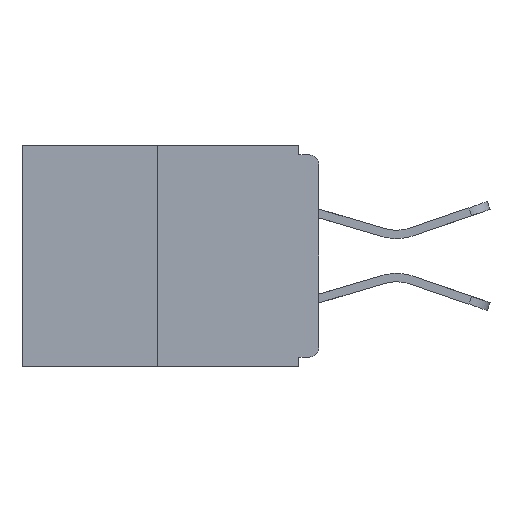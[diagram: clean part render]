
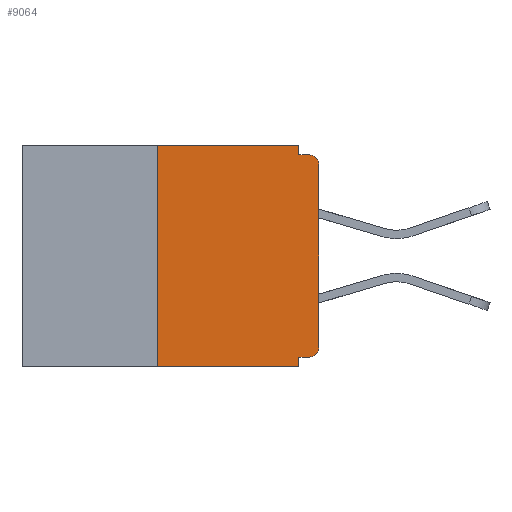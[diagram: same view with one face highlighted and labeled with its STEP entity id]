
A CAD part, left-side view. The second image highlights one B-rep face of the part: STEP entity #9064.
In plain terms, the highlighted planar face has unit normal (-1, 0, 0).
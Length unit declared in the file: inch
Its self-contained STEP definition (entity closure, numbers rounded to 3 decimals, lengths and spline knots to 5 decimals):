
#79 = VECTOR ( 'NONE', #12660, 39.37008 ) ;
#108 = VERTEX_POINT ( 'NONE', #13360 ) ;
#824 = EDGE_CURVE ( 'NONE', #8475, #1453, #8395, .T. ) ;
#834 = VERTEX_POINT ( 'NONE', #13838 ) ;
#1170 = AXIS2_PLACEMENT_3D ( 'NONE', #12093, #9109, #7771 ) ;
#1222 = DIRECTION ( 'NONE',  ( 0., 0., -1. ) ) ;
#1316 = LINE ( 'NONE', #3704, #11945 ) ;
#1453 = VERTEX_POINT ( 'NONE', #11990 ) ;
#1483 = LINE ( 'NONE', #13181, #8561 ) ;
#1779 = VERTEX_POINT ( 'NONE', #2282 ) ;
#2138 = EDGE_CURVE ( 'NONE', #9694, #13709, #9196, .T. ) ;
#2282 = CARTESIAN_POINT ( 'NONE',  ( 0., 0.031, 0. ) ) ;
#2665 = CARTESIAN_POINT ( 'NONE',  ( 0., 0.25, 0. ) ) ;
#2887 = VERTEX_POINT ( 'NONE', #2665 ) ;
#3097 = CIRCLE ( 'NONE', #13831, 0.015 ) ;
#3277 = EDGE_CURVE ( 'NONE', #10018, #8149, #6022, .T. ) ;
#3427 = LINE ( 'NONE', #7977, #13079 ) ;
#3610 = DIRECTION ( 'NONE',  ( -1., 0., 0. ) ) ;
#3704 = CARTESIAN_POINT ( 'NONE',  ( 0., 0.46, 0. ) ) ;
#4407 = CARTESIAN_POINT ( 'NONE',  ( 0., 0.031, -0.343 ) ) ;
#4533 = EDGE_CURVE ( 'NONE', #1779, #9694, #1483, .T. ) ;
#4693 = CARTESIAN_POINT ( 'NONE',  ( 0., 0., -0.03 ) ) ;
#4867 = DIRECTION ( 'NONE',  ( 0., 0., -1. ) ) ;
#5077 = ORIENTED_EDGE ( 'NONE', *, *, #824, .T. ) ;
#5130 = EDGE_CURVE ( 'NONE', #834, #10018, #3097, .T. ) ;
#5134 = CARTESIAN_POINT ( 'NONE',  ( 0., 0., -0.015 ) ) ;
#5145 = VECTOR ( 'NONE', #9404, 39.37008 ) ;
#5468 = LINE ( 'NONE', #6390, #8571 ) ;
#5552 = CARTESIAN_POINT ( 'NONE',  ( 0., 0.031, -0.015 ) ) ;
#5947 = DIRECTION ( 'NONE',  ( 0., 0., 1. ) ) ;
#6022 = LINE ( 'NONE', #10296, #7125 ) ;
#6390 = CARTESIAN_POINT ( 'NONE',  ( 0., 0., -0.328 ) ) ;
#6522 = EDGE_CURVE ( 'NONE', #8149, #13709, #8382, .T. ) ;
#6644 = DIRECTION ( 'NONE',  ( 0., 0., -1. ) ) ;
#6874 = EDGE_CURVE ( 'NONE', #2887, #1779, #1316, .T. ) ;
#6895 = EDGE_CURVE ( 'NONE', #8475, #2887, #3427, .T. ) ;
#7092 = ORIENTED_EDGE ( 'NONE', *, *, #5130, .T. ) ;
#7105 = DIRECTION ( 'NONE',  ( -1., 0., 0. ) ) ;
#7125 = VECTOR ( 'NONE', #5947, 39.37008 ) ;
#7231 = ORIENTED_EDGE ( 'NONE', *, *, #6874, .F. ) ;
#7608 = ORIENTED_EDGE ( 'NONE', *, *, #4533, .F. ) ;
#7771 = DIRECTION ( 'NONE',  ( 0., 0., -1. ) ) ;
#7909 = FACE_OUTER_BOUND ( 'NONE', #12830, .T. ) ;
#7945 = CARTESIAN_POINT ( 'NONE',  ( 0., 0.015, -0.313 ) ) ;
#7977 = CARTESIAN_POINT ( 'NONE',  ( 0., 0.25, 0. ) ) ;
#8149 = VERTEX_POINT ( 'NONE', #4693 ) ;
#8271 = CARTESIAN_POINT ( 'NONE',  ( 0., 0.25, -0.343 ) ) ;
#8382 = CIRCLE ( 'NONE', #11055, 0.015 ) ;
#8395 = LINE ( 'NONE', #10496, #79 ) ;
#8475 = VERTEX_POINT ( 'NONE', #8271 ) ;
#8561 = VECTOR ( 'NONE', #11976, 39.37008 ) ;
#8571 = VECTOR ( 'NONE', #10665, 39.37008 ) ;
#9064 = ADVANCED_FACE ( 'NONE', ( #7909 ), #9875, .F. ) ;
#9109 = DIRECTION ( 'NONE',  ( 1., 0., 0. ) ) ;
#9196 = LINE ( 'NONE', #5134, #5145 ) ;
#9392 = ORIENTED_EDGE ( 'NONE', *, *, #6895, .F. ) ;
#9404 = DIRECTION ( 'NONE',  ( 0., -1., 0. ) ) ;
#9694 = VERTEX_POINT ( 'NONE', #5552 ) ;
#9875 = PLANE ( 'NONE',  #1170 ) ;
#10010 = ORIENTED_EDGE ( 'NONE', *, *, #10137, .F. ) ;
#10018 = VERTEX_POINT ( 'NONE', #12684 ) ;
#10080 = DIRECTION ( 'NONE',  ( 0., 0., 1. ) ) ;
#10137 = EDGE_CURVE ( 'NONE', #834, #108, #5468, .T. ) ;
#10148 = VECTOR ( 'NONE', #6644, 39.37008 ) ;
#10296 = CARTESIAN_POINT ( 'NONE',  ( 0., 0., 0. ) ) ;
#10496 = CARTESIAN_POINT ( 'NONE',  ( 0., 0.46, -0.343 ) ) ;
#10508 = ORIENTED_EDGE ( 'NONE', *, *, #3277, .T. ) ;
#10665 = DIRECTION ( 'NONE',  ( 0., 1., 0. ) ) ;
#10838 = LINE ( 'NONE', #4407, #10148 ) ;
#10885 = CARTESIAN_POINT ( 'NONE',  ( 0., 0.015, -0.03 ) ) ;
#10898 = ORIENTED_EDGE ( 'NONE', *, *, #6522, .T. ) ;
#11055 = AXIS2_PLACEMENT_3D ( 'NONE', #10885, #3610, #1222 ) ;
#11111 = EDGE_CURVE ( 'NONE', #108, #1453, #10838, .T. ) ;
#11709 = ORIENTED_EDGE ( 'NONE', *, *, #2138, .F. ) ;
#11945 = VECTOR ( 'NONE', #12165, 39.37008 ) ;
#11976 = DIRECTION ( 'NONE',  ( 0., 0., -1. ) ) ;
#11990 = CARTESIAN_POINT ( 'NONE',  ( 0., 0.031, -0.343 ) ) ;
#12093 = CARTESIAN_POINT ( 'NONE',  ( 0., 0.46, 0. ) ) ;
#12165 = DIRECTION ( 'NONE',  ( 0., -1., 0. ) ) ;
#12353 = CARTESIAN_POINT ( 'NONE',  ( 0., 0.015, -0.015 ) ) ;
#12660 = DIRECTION ( 'NONE',  ( 0., -1., 0. ) ) ;
#12684 = CARTESIAN_POINT ( 'NONE',  ( 0., 0., -0.313 ) ) ;
#12830 = EDGE_LOOP ( 'NONE', ( #7231, #9392, #5077, #13628, #10010, #7092, #10508, #10898, #11709, #7608 ) ) ;
#13079 = VECTOR ( 'NONE', #10080, 39.37008 ) ;
#13181 = CARTESIAN_POINT ( 'NONE',  ( 0., 0.031, 0. ) ) ;
#13360 = CARTESIAN_POINT ( 'NONE',  ( 0., 0.031, -0.328 ) ) ;
#13628 = ORIENTED_EDGE ( 'NONE', *, *, #11111, .F. ) ;
#13709 = VERTEX_POINT ( 'NONE', #12353 ) ;
#13831 = AXIS2_PLACEMENT_3D ( 'NONE', #7945, #7105, #4867 ) ;
#13838 = CARTESIAN_POINT ( 'NONE',  ( 0., 0.015, -0.328 ) ) ;
